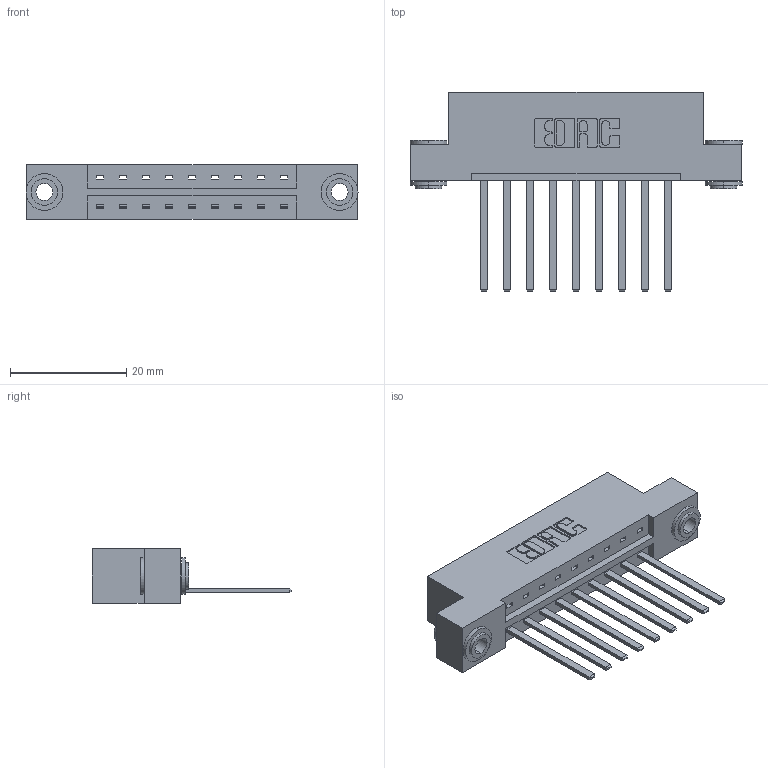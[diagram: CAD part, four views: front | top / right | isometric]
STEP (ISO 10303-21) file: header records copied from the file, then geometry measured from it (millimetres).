
FILE_DESCRIPTION (( 'STEP AP203' ), '1' );
FILE_NAME ('333-009-544-103.STEP', '2018-07-31T22:36:36', ( '' ), ( '' ), 'SwSTEP 2.0', 'SolidWorks 2016', '' );
FILE_SCHEMA (( 'CONFIG_CONTROL_DESIGN' ));
Length unit declared in the file: inch
Products named in the file (4): 333 Part_Flush - .156 Dia - TH; 345-292-001_345-293-144; 345-250-002_345-250-002-102; 333-009-544-103
Assembly tree (12 placements, depth 2):
  333-009-544-103
    333 Part_Flush - .156 Dia - TH
    345-292-001_345-293-144  x9
    345-250-002_345-250-002-102  x2
Bounding box: 57.2 x 34.3 x 9.4 mm (x, y, z)
Volume: 5595.8 mm3; surface area: 6405.1 mm2
Topology: 12 solids, 12 shells, 620 faces, 1809 edges, 1190 vertices
Faces by surface type: plane 422, cylinder 190, cone 8
Entity records: 10236 total; most frequent: CARTESIAN_POINT 1748, ORIENTED_EDGE 1686, DIRECTION 1571, EDGE_CURVE 843, VECTOR 695, LINE 695, VERTEX_POINT 558, AXIS2_PLACEMENT_3D 438
